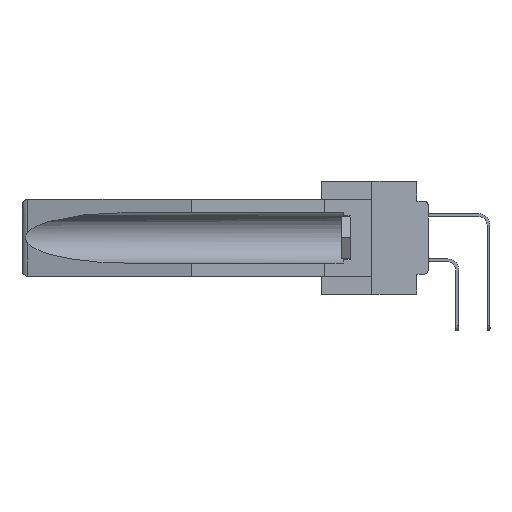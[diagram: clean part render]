
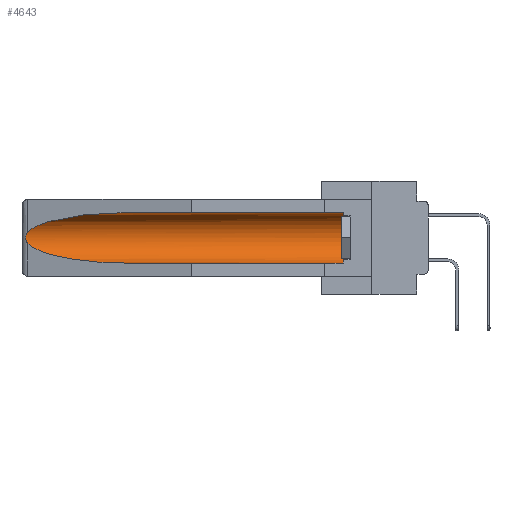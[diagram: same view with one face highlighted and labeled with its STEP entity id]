
A CAD part, left-side view. The second image highlights one B-rep face of the part: STEP entity #4643.
In plain terms, the highlighted cylindrical face has radius 2.857 mm (diameter 5.715 mm), a partial arc.
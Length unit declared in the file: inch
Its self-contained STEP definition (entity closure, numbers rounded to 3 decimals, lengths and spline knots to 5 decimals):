
#235 = EDGE_CURVE ( 'NONE', #31400, #4098, #330, .T. ) ;
#330 = B_SPLINE_CURVE_WITH_KNOTS ( 'NONE', 3,
 ( #13903, #33074, #19229, #8193, #30379, #13794, #22116, #22246, #33310, #16669 ),
 .UNSPECIFIED., .F., .F.,
 ( 4, 2, 2, 2, 4 ),
 ( 0., 0.00029, 0.00058, 0.00087, 0.00117 ),
 .UNSPECIFIED. ) ;
#489 = CARTESIAN_POINT ( 'NONE',  ( 0.155, 1.07973, -0.284 ) ) ;
#977 = DIRECTION ( 'NONE',  ( 0., -1., 0. ) ) ;
#1719 = CARTESIAN_POINT ( 'NONE',  ( 0.26537, 1.52718, -0.14972 ) ) ;
#3019 = DIRECTION ( 'NONE',  ( 0., 0., 1. ) ) ;
#3833 = AXIS2_PLACEMENT_3D ( 'NONE', #6062, #977, #25564 ) ;
#4098 = VERTEX_POINT ( 'NONE', #27761 ) ;
#4104 =( BOUNDED_CURVE ( )  B_SPLINE_CURVE ( 3, ( #21871, #21217, #24666, #27471 ),
 .UNSPECIFIED., .F., .F. ) 
 B_SPLINE_CURVE_WITH_KNOTS ( ( 4, 4 ),
 ( 4.71239, 6.08839 ),
 .UNSPECIFIED. ) 
 CURVE ( )  GEOMETRIC_REPRESENTATION_ITEM ( )  RATIONAL_B_SPLINE_CURVE ( ( 1., 0.848, 0.848, 1. ) ) 
 REPRESENTATION_ITEM ( '' )  );
#4643 = ADVANCED_FACE ( 'NONE', ( #5259 ), #10458, .F. ) ;
#5257 = EDGE_CURVE ( 'NONE', #27767, #31400, #4104, .T. ) ;
#5259 = FACE_OUTER_BOUND ( 'NONE', #30458, .T. ) ;
#5641 = EDGE_CURVE ( 'NONE', #4098, #23673, #17010, .T. ) ;
#6062 = CARTESIAN_POINT ( 'NONE',  ( 0.155, 0.126, -0.1715 ) ) ;
#8193 = CARTESIAN_POINT ( 'NONE',  ( 0.2673, 1.5327, -0.16383 ) ) ;
#8553 = VERTEX_POINT ( 'NONE', #13677 ) ;
#10378 = CARTESIAN_POINT ( 'NONE',  ( 0.155, 0.126, -0.059 ) ) ;
#10458 = CYLINDRICAL_SURFACE ( 'NONE', #31043, 0.1125 ) ;
#10572 = CIRCLE ( 'NONE', #3833, 0.1125 ) ;
#12956 = EDGE_CURVE ( 'NONE', #8553, #23673, #29230, .T. ) ;
#13133 = EDGE_CURVE ( 'NONE', #8553, #18330, #10572, .T. ) ;
#13442 = VECTOR ( 'NONE', #33297, 39.37008 ) ;
#13677 = CARTESIAN_POINT ( 'NONE',  ( 0.155, 0.126, -0.284 ) ) ;
#13794 = CARTESIAN_POINT ( 'NONE',  ( 0.2675, 1.53308, -0.17534 ) ) ;
#13903 = CARTESIAN_POINT ( 'NONE',  ( 0.26537, 1.52718, -0.14972 ) ) ;
#14313 = LINE ( 'NONE', #17006, #13442 ) ;
#16280 = ORIENTED_EDGE ( 'NONE', *, *, #28255, .T. ) ;
#16669 = CARTESIAN_POINT ( 'NONE',  ( 0.26537, 1.52718, -0.19328 ) ) ;
#16954 = CARTESIAN_POINT ( 'NONE',  ( 0.26537, 1.52718, -0.19328 ) ) ;
#17006 = CARTESIAN_POINT ( 'NONE',  ( 0.155, -0.30754, -0.059 ) ) ;
#17010 =( BOUNDED_CURVE ( )  B_SPLINE_CURVE ( 3, ( #16954, #25323, #25191, #489 ),
 .UNSPECIFIED., .F., .F. ) 
 B_SPLINE_CURVE_WITH_KNOTS ( ( 4, 4 ),
 ( 0.1948, 1.5708 ),
 .UNSPECIFIED. ) 
 CURVE ( )  GEOMETRIC_REPRESENTATION_ITEM ( )  RATIONAL_B_SPLINE_CURVE ( ( 1., 0.848, 0.848, 1. ) ) 
 REPRESENTATION_ITEM ( '' )  );
#17171 = CARTESIAN_POINT ( 'NONE',  ( 0.155, -0.30754, -0.1715 ) ) ;
#17375 = ORIENTED_EDGE ( 'NONE', *, *, #12956, .F. ) ;
#18330 = VERTEX_POINT ( 'NONE', #10378 ) ;
#19229 = CARTESIAN_POINT ( 'NONE',  ( 0.26654, 1.53092, -0.15636 ) ) ;
#19813 = DIRECTION ( 'NONE',  ( 0., 1., 0. ) ) ;
#20559 = CARTESIAN_POINT ( 'NONE',  ( 0.155, 1.07973, -0.059 ) ) ;
#21217 = CARTESIAN_POINT ( 'NONE',  ( 0.21114, 1.30732, -0.059 ) ) ;
#21871 = CARTESIAN_POINT ( 'NONE',  ( 0.155, 1.07973, -0.059 ) ) ;
#22116 = CARTESIAN_POINT ( 'NONE',  ( 0.2673, 1.53269, -0.17917 ) ) ;
#22246 = CARTESIAN_POINT ( 'NONE',  ( 0.26655, 1.53094, -0.18657 ) ) ;
#22831 = ORIENTED_EDGE ( 'NONE', *, *, #235, .T. ) ;
#23668 = CARTESIAN_POINT ( 'NONE',  ( 0.155, 1.07973, -0.284 ) ) ;
#23673 = VERTEX_POINT ( 'NONE', #23668 ) ;
#23881 = ORIENTED_EDGE ( 'NONE', *, *, #13133, .T. ) ;
#24574 = ORIENTED_EDGE ( 'NONE', *, *, #5257, .T. ) ;
#24666 = CARTESIAN_POINT ( 'NONE',  ( 0.25451, 1.48313, -0.09465 ) ) ;
#25101 = ORIENTED_EDGE ( 'NONE', *, *, #5641, .T. ) ;
#25191 = CARTESIAN_POINT ( 'NONE',  ( 0.21114, 1.30732, -0.284 ) ) ;
#25323 = CARTESIAN_POINT ( 'NONE',  ( 0.25451, 1.48313, -0.24835 ) ) ;
#25400 = DIRECTION ( 'NONE',  ( 0., 1., 0. ) ) ;
#25564 = DIRECTION ( 'NONE',  ( 0., 0., 1. ) ) ;
#27471 = CARTESIAN_POINT ( 'NONE',  ( 0.26537, 1.52718, -0.14972 ) ) ;
#27761 = CARTESIAN_POINT ( 'NONE',  ( 0.26537, 1.52718, -0.19328 ) ) ;
#27767 = VERTEX_POINT ( 'NONE', #20559 ) ;
#28255 = EDGE_CURVE ( 'NONE', #18330, #27767, #14313, .T. ) ;
#29230 = LINE ( 'NONE', #33889, #35788 ) ;
#30379 = CARTESIAN_POINT ( 'NONE',  ( 0.2675, 1.53308, -0.16763 ) ) ;
#30458 = EDGE_LOOP ( 'NONE', ( #24574, #22831, #25101, #17375, #23881, #16280 ) ) ;
#31043 = AXIS2_PLACEMENT_3D ( 'NONE', #17171, #25400, #3019 ) ;
#31400 = VERTEX_POINT ( 'NONE', #1719 ) ;
#33074 = CARTESIAN_POINT ( 'NONE',  ( 0.26597, 1.52961, -0.15275 ) ) ;
#33297 = DIRECTION ( 'NONE',  ( 0., 1., 0. ) ) ;
#33310 = CARTESIAN_POINT ( 'NONE',  ( 0.26597, 1.5296, -0.19026 ) ) ;
#33889 = CARTESIAN_POINT ( 'NONE',  ( 0.155, -0.30754, -0.284 ) ) ;
#35788 = VECTOR ( 'NONE', #19813, 39.37008 ) ;
